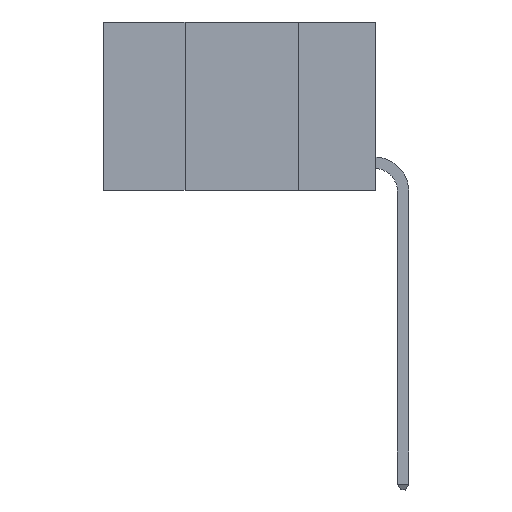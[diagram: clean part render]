
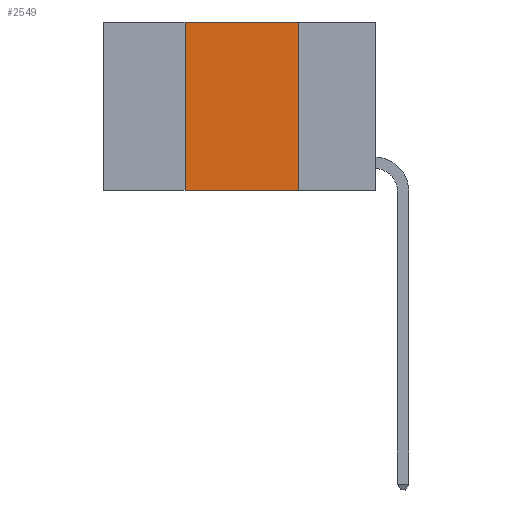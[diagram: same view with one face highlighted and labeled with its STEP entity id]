
A CAD part, left-side view. The second image highlights one B-rep face of the part: STEP entity #2549.
In plain terms, the highlighted planar face has unit normal (-1, 0, 0).
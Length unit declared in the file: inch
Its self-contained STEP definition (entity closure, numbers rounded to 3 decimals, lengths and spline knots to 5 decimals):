
#834 = EDGE_CURVE ( 'NONE', #19675, #4958, #20641, .T. ) ;
#1884 = ORIENTED_EDGE ( 'NONE', *, *, #834, .F. ) ;
#2294 = CARTESIAN_POINT ( 'NONE',  ( 0., 0.42, 0. ) ) ;
#2549 = ADVANCED_FACE ( 'NONE', ( #3575 ), #16429, .F. ) ;
#2601 = CARTESIAN_POINT ( 'NONE',  ( 0., 0.42, 0. ) ) ;
#2933 = CARTESIAN_POINT ( 'NONE',  ( 0., 0.6, 0. ) ) ;
#3173 = CARTESIAN_POINT ( 'NONE',  ( 0., 0.42, -0.37 ) ) ;
#3575 = FACE_OUTER_BOUND ( 'NONE', #19213, .T. ) ;
#4958 = VERTEX_POINT ( 'NONE', #2294 ) ;
#5507 = ORIENTED_EDGE ( 'NONE', *, *, #13047, .F. ) ;
#6594 = ORIENTED_EDGE ( 'NONE', *, *, #12240, .T. ) ;
#6923 = DIRECTION ( 'NONE',  ( 0., 0., 1. ) ) ;
#7414 = LINE ( 'NONE', #10399, #19525 ) ;
#7866 = CARTESIAN_POINT ( 'NONE',  ( 0., 0.6, -0.37 ) ) ;
#8205 = DIRECTION ( 'NONE',  ( 1., 0., 0. ) ) ;
#9293 = VERTEX_POINT ( 'NONE', #14685 ) ;
#10399 = CARTESIAN_POINT ( 'NONE',  ( 0., 0.6, 0. ) ) ;
#11688 = VECTOR ( 'NONE', #18055, 39.37008 ) ;
#12060 = DIRECTION ( 'NONE',  ( 0., -1., 0. ) ) ;
#12240 = EDGE_CURVE ( 'NONE', #19675, #17287, #17081, .T. ) ;
#12722 = VECTOR ( 'NONE', #17711, 39.37008 ) ;
#13047 = EDGE_CURVE ( 'NONE', #9293, #17287, #20921, .T. ) ;
#14380 = ORIENTED_EDGE ( 'NONE', *, *, #18537, .F. ) ;
#14685 = CARTESIAN_POINT ( 'NONE',  ( 0., 0.17, 0. ) ) ;
#16429 = PLANE ( 'NONE',  #21437 ) ;
#16492 = CARTESIAN_POINT ( 'NONE',  ( 0., 0.17, 0. ) ) ;
#17081 = LINE ( 'NONE', #7866, #12722 ) ;
#17243 = CARTESIAN_POINT ( 'NONE',  ( 0., 0.17, -0.37 ) ) ;
#17287 = VERTEX_POINT ( 'NONE', #17243 ) ;
#17711 = DIRECTION ( 'NONE',  ( 0., -1., 0. ) ) ;
#18055 = DIRECTION ( 'NONE',  ( 0., 0., -1. ) ) ;
#18537 = EDGE_CURVE ( 'NONE', #4958, #9293, #7414, .T. ) ;
#19213 = EDGE_LOOP ( 'NONE', ( #5507, #14380, #1884, #6594 ) ) ;
#19525 = VECTOR ( 'NONE', #12060, 39.37008 ) ;
#19675 = VERTEX_POINT ( 'NONE', #3173 ) ;
#19709 = DIRECTION ( 'NONE',  ( 0., 0., -1. ) ) ;
#20641 = LINE ( 'NONE', #2601, #21167 ) ;
#20921 = LINE ( 'NONE', #16492, #11688 ) ;
#21167 = VECTOR ( 'NONE', #6923, 39.37008 ) ;
#21437 = AXIS2_PLACEMENT_3D ( 'NONE', #2933, #8205, #19709 ) ;
